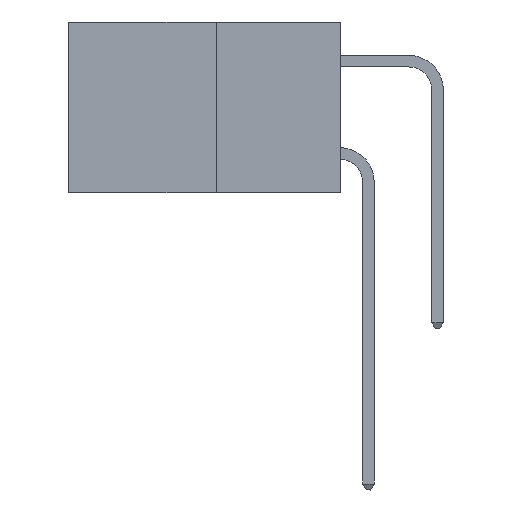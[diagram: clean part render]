
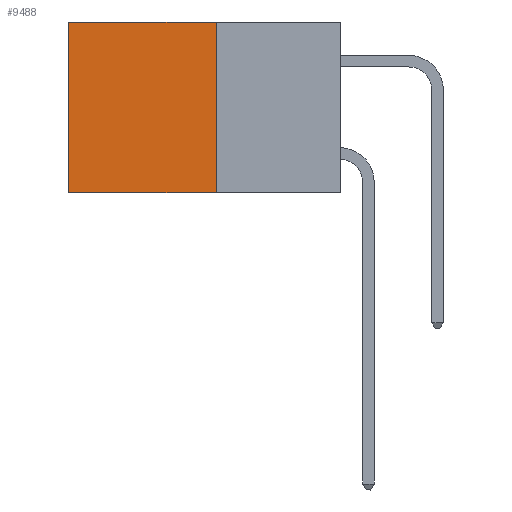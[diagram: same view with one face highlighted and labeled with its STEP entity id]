
A CAD part, left-side view. The second image highlights one B-rep face of the part: STEP entity #9488.
In plain terms, the highlighted planar face has unit normal (-1, 0, 0).
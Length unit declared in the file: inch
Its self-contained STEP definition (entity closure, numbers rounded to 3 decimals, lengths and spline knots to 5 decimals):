
#478 = EDGE_CURVE ( 'NONE', #12983, #18408, #15454, .T. ) ;
#924 = EDGE_LOOP ( 'NONE', ( #18149, #16606, #14457, #18721 ) ) ;
#1056 = FACE_OUTER_BOUND ( 'NONE', #924, .T. ) ;
#1512 = CARTESIAN_POINT ( 'NONE',  ( 0.277, 0.27, -0.37 ) ) ;
#2036 = AXIS2_PLACEMENT_3D ( 'NONE', #15172, #18510, #8742 ) ;
#3364 = CARTESIAN_POINT ( 'NONE',  ( 0.277, 0.59, -0.37 ) ) ;
#4153 = DIRECTION ( 'NONE',  ( 0., 0., -1. ) ) ;
#4889 = VERTEX_POINT ( 'NONE', #7567 ) ;
#5012 = VECTOR ( 'NONE', #20011, 39.37008 ) ;
#5742 = VECTOR ( 'NONE', #6593, 39.37008 ) ;
#6593 = DIRECTION ( 'NONE',  ( 0., 0., -1. ) ) ;
#6870 = VECTOR ( 'NONE', #9008, 39.37008 ) ;
#7567 = CARTESIAN_POINT ( 'NONE',  ( 0.277, 0.59, 0. ) ) ;
#7804 = CARTESIAN_POINT ( 'NONE',  ( 0.277, 0.27, -0.37 ) ) ;
#8742 = DIRECTION ( 'NONE',  ( 0., 0., -1. ) ) ;
#9008 = DIRECTION ( 'NONE',  ( 0., 1., 0. ) ) ;
#9262 = CARTESIAN_POINT ( 'NONE',  ( 0.277, 0.27, 0. ) ) ;
#9362 = LINE ( 'NONE', #16764, #5012 ) ;
#9464 = EDGE_CURVE ( 'NONE', #12624, #4889, #9362, .T. ) ;
#9488 = ADVANCED_FACE ( 'NONE', ( #1056 ), #13500, .F. ) ;
#10080 = CARTESIAN_POINT ( 'NONE',  ( 0.277, 0.27, -0.37 ) ) ;
#11961 = LINE ( 'NONE', #13867, #16835 ) ;
#12624 = VERTEX_POINT ( 'NONE', #9262 ) ;
#12983 = VERTEX_POINT ( 'NONE', #10080 ) ;
#13500 = PLANE ( 'NONE',  #2036 ) ;
#13867 = CARTESIAN_POINT ( 'NONE',  ( 0.277, 0.59, -0.37 ) ) ;
#14457 = ORIENTED_EDGE ( 'NONE', *, *, #18888, .F. ) ;
#14844 = LINE ( 'NONE', #1512, #5742 ) ;
#15172 = CARTESIAN_POINT ( 'NONE',  ( 0.277, 0.27, -0.37 ) ) ;
#15342 = EDGE_CURVE ( 'NONE', #4889, #18408, #11961, .T. ) ;
#15454 = LINE ( 'NONE', #7804, #6870 ) ;
#16606 = ORIENTED_EDGE ( 'NONE', *, *, #478, .F. ) ;
#16764 = CARTESIAN_POINT ( 'NONE',  ( 0.277, 0.27, 0. ) ) ;
#16835 = VECTOR ( 'NONE', #4153, 39.37008 ) ;
#18149 = ORIENTED_EDGE ( 'NONE', *, *, #15342, .T. ) ;
#18408 = VERTEX_POINT ( 'NONE', #3364 ) ;
#18510 = DIRECTION ( 'NONE',  ( 1., 0., 0. ) ) ;
#18721 = ORIENTED_EDGE ( 'NONE', *, *, #9464, .T. ) ;
#18888 = EDGE_CURVE ( 'NONE', #12624, #12983, #14844, .T. ) ;
#20011 = DIRECTION ( 'NONE',  ( 0., 1., 0. ) ) ;
